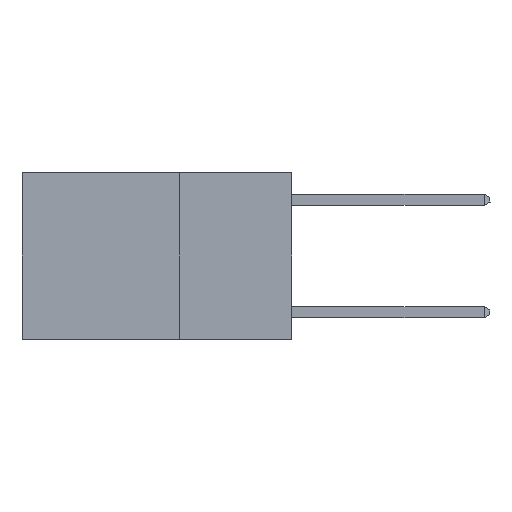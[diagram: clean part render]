
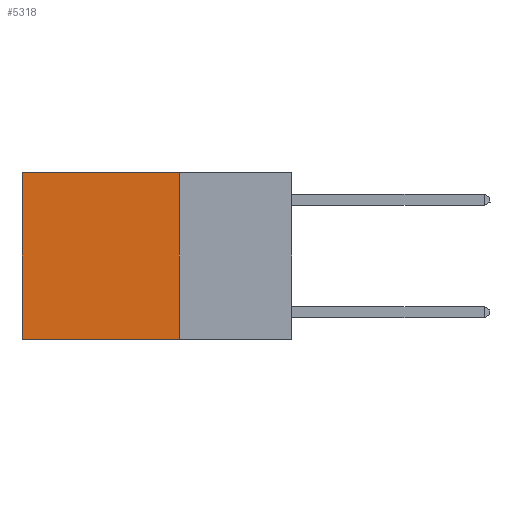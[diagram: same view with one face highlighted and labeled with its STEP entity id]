
A CAD part, left-side view. The second image highlights one B-rep face of the part: STEP entity #5318.
In plain terms, the highlighted planar face has unit normal (-1, 0, 0).
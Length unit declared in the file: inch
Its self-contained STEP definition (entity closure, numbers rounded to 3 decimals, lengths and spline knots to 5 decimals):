
#19 = DIRECTION ( 'NONE',  ( 0., 1., 0. ) ) ;
#21 = AXIS2_PLACEMENT_3D ( 'NONE', #9226, #2313, #11973 ) ;
#565 = VERTEX_POINT ( 'NONE', #11939 ) ;
#652 = ORIENTED_EDGE ( 'NONE', *, *, #2814, .F. ) ;
#873 = PLANE ( 'NONE',  #21 ) ;
#1908 = EDGE_CURVE ( 'NONE', #7808, #12177, #6473, .T. ) ;
#2313 = DIRECTION ( 'NONE',  ( 1., 0., 0. ) ) ;
#2814 = EDGE_CURVE ( 'NONE', #17028, #12177, #5780, .T. ) ;
#3877 = LINE ( 'NONE', #14682, #7178 ) ;
#5318 = ADVANCED_FACE ( 'NONE', ( #6090 ), #873, .F. ) ;
#5340 = EDGE_LOOP ( 'NONE', ( #12242, #652, #11948, #8861 ) ) ;
#5780 = LINE ( 'NONE', #7167, #16102 ) ;
#5836 = EDGE_CURVE ( 'NONE', #565, #17028, #3877, .T. ) ;
#6090 = FACE_OUTER_BOUND ( 'NONE', #5340, .T. ) ;
#6473 = LINE ( 'NONE', #15702, #16761 ) ;
#6631 = CARTESIAN_POINT ( 'NONE',  ( 0.2625, 0.6, -0.37 ) ) ;
#7057 = CARTESIAN_POINT ( 'NONE',  ( 0.2625, 0.25, 0. ) ) ;
#7167 = CARTESIAN_POINT ( 'NONE',  ( 0.2625, 0.25, -0.37 ) ) ;
#7178 = VECTOR ( 'NONE', #7925, 39.37008 ) ;
#7666 = DIRECTION ( 'NONE',  ( 0., 0., -1. ) ) ;
#7808 = VERTEX_POINT ( 'NONE', #11610 ) ;
#7925 = DIRECTION ( 'NONE',  ( 0., 0., -1. ) ) ;
#8485 = DIRECTION ( 'NONE',  ( 0., 1., 0. ) ) ;
#8861 = ORIENTED_EDGE ( 'NONE', *, *, #12401, .T. ) ;
#9226 = CARTESIAN_POINT ( 'NONE',  ( 0.2625, 0.25, 0. ) ) ;
#11610 = CARTESIAN_POINT ( 'NONE',  ( 0.2625, 0.6, 0. ) ) ;
#11939 = CARTESIAN_POINT ( 'NONE',  ( 0.2625, 0.25, 0. ) ) ;
#11948 = ORIENTED_EDGE ( 'NONE', *, *, #5836, .F. ) ;
#11973 = DIRECTION ( 'NONE',  ( 0., 0., -1. ) ) ;
#12177 = VERTEX_POINT ( 'NONE', #6631 ) ;
#12242 = ORIENTED_EDGE ( 'NONE', *, *, #1908, .T. ) ;
#12386 = CARTESIAN_POINT ( 'NONE',  ( 0.2625, 0.25, -0.37 ) ) ;
#12401 = EDGE_CURVE ( 'NONE', #565, #7808, #12914, .T. ) ;
#12476 = VECTOR ( 'NONE', #19, 39.37008 ) ;
#12914 = LINE ( 'NONE', #7057, #12476 ) ;
#14682 = CARTESIAN_POINT ( 'NONE',  ( 0.2625, 0.25, 0. ) ) ;
#15702 = CARTESIAN_POINT ( 'NONE',  ( 0.2625, 0.6, 0. ) ) ;
#16102 = VECTOR ( 'NONE', #8485, 39.37008 ) ;
#16761 = VECTOR ( 'NONE', #7666, 39.37008 ) ;
#17028 = VERTEX_POINT ( 'NONE', #12386 ) ;
